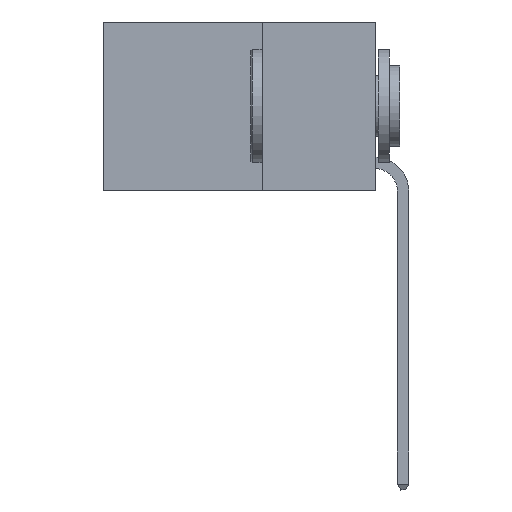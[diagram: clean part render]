
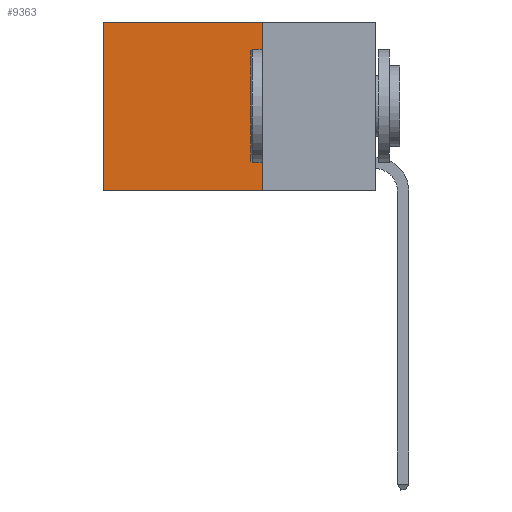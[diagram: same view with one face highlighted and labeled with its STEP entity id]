
A CAD part, left-side view. The second image highlights one B-rep face of the part: STEP entity #9363.
In plain terms, the highlighted planar face has unit normal (-1, 0, 0).
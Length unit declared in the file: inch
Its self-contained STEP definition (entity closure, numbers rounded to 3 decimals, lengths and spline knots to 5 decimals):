
#363 = EDGE_CURVE ( 'NONE', #22062, #6080, #24423, .T. ) ;
#917 = DIRECTION ( 'NONE',  ( 0., 0., -1. ) ) ;
#2730 = CARTESIAN_POINT ( 'NONE',  ( 0.2625, 0.25, -0.37 ) ) ;
#3121 = DIRECTION ( 'NONE',  ( 0., 0., -1. ) ) ;
#3252 = CARTESIAN_POINT ( 'NONE',  ( 0.2625, 0.25, 0. ) ) ;
#3387 = CARTESIAN_POINT ( 'NONE',  ( 0.2625, 0.6, 0. ) ) ;
#4101 = EDGE_CURVE ( 'NONE', #6080, #20758, #14102, .T. ) ;
#4351 = VECTOR ( 'NONE', #16712, 39.37008 ) ;
#4361 = CARTESIAN_POINT ( 'NONE',  ( 0.2625, 0.6, 0. ) ) ;
#6080 = VERTEX_POINT ( 'NONE', #3387 ) ;
#7975 = EDGE_LOOP ( 'NONE', ( #19219, #22377, #15311, #12705 ) ) ;
#9363 = ADVANCED_FACE ( 'NONE', ( #12899 ), #13029, .F. ) ;
#10144 = VECTOR ( 'NONE', #917, 39.37008 ) ;
#10613 = CARTESIAN_POINT ( 'NONE',  ( 0.2625, 0.25, 0. ) ) ;
#10910 = VECTOR ( 'NONE', #21931, 39.37008 ) ;
#12705 = ORIENTED_EDGE ( 'NONE', *, *, #363, .T. ) ;
#12899 = FACE_OUTER_BOUND ( 'NONE', #7975, .T. ) ;
#13029 = PLANE ( 'NONE',  #14486 ) ;
#14102 = LINE ( 'NONE', #4361, #22750 ) ;
#14297 = VERTEX_POINT ( 'NONE', #2730 ) ;
#14336 = CARTESIAN_POINT ( 'NONE',  ( 0.2625, 0.25, -0.37 ) ) ;
#14486 = AXIS2_PLACEMENT_3D ( 'NONE', #3252, #20979, #3121 ) ;
#15311 = ORIENTED_EDGE ( 'NONE', *, *, #17423, .F. ) ;
#16055 = EDGE_CURVE ( 'NONE', #14297, #20758, #23753, .T. ) ;
#16712 = DIRECTION ( 'NONE',  ( 0., 1., 0. ) ) ;
#17423 = EDGE_CURVE ( 'NONE', #22062, #14297, #22581, .T. ) ;
#17892 = DIRECTION ( 'NONE',  ( 0., 0., -1. ) ) ;
#19219 = ORIENTED_EDGE ( 'NONE', *, *, #4101, .T. ) ;
#19853 = CARTESIAN_POINT ( 'NONE',  ( 0.2625, 0.6, -0.37 ) ) ;
#20758 = VERTEX_POINT ( 'NONE', #19853 ) ;
#20979 = DIRECTION ( 'NONE',  ( 1., 0., 0. ) ) ;
#21931 = DIRECTION ( 'NONE',  ( 0., 1., 0. ) ) ;
#22062 = VERTEX_POINT ( 'NONE', #22098 ) ;
#22098 = CARTESIAN_POINT ( 'NONE',  ( 0.2625, 0.25, 0. ) ) ;
#22377 = ORIENTED_EDGE ( 'NONE', *, *, #16055, .F. ) ;
#22581 = LINE ( 'NONE', #24650, #10144 ) ;
#22750 = VECTOR ( 'NONE', #17892, 39.37008 ) ;
#23753 = LINE ( 'NONE', #14336, #10910 ) ;
#24423 = LINE ( 'NONE', #10613, #4351 ) ;
#24650 = CARTESIAN_POINT ( 'NONE',  ( 0.2625, 0.25, 0. ) ) ;
